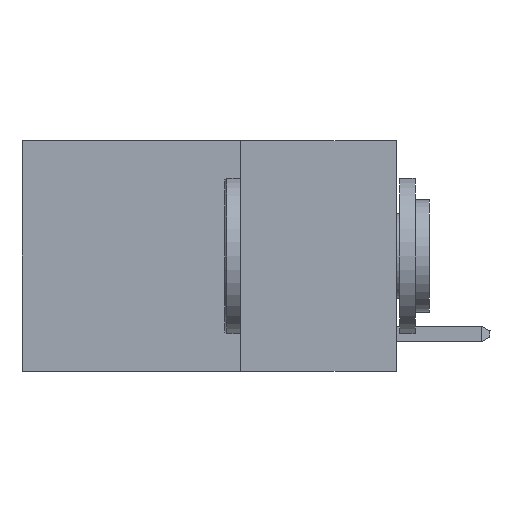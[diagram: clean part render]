
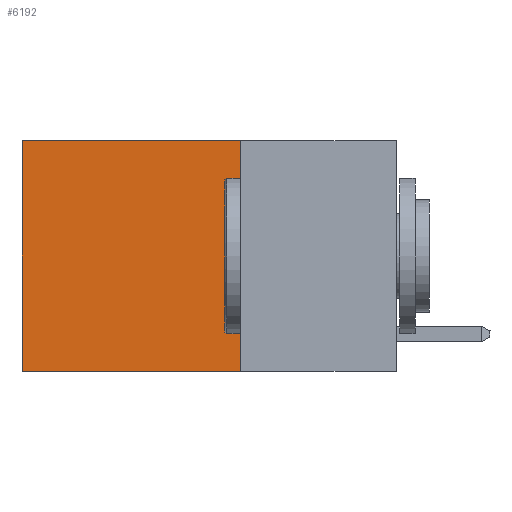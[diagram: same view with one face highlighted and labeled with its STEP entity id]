
A CAD part, left-side view. The second image highlights one B-rep face of the part: STEP entity #6192.
In plain terms, the highlighted planar face has unit normal (-1, 0, 0).
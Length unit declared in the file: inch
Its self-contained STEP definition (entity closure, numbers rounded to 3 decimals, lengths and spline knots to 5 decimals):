
#1 = DIRECTION ( 'NONE',  ( 0., 1., 0. ) ) ;
#405 = CARTESIAN_POINT ( 'NONE',  ( 0.2625, 0.6, 0. ) ) ;
#1059 = DIRECTION ( 'NONE',  ( 0., 0., -1. ) ) ;
#1090 = EDGE_CURVE ( 'NONE', #13211, #1268, #5037, .T. ) ;
#1151 = EDGE_CURVE ( 'NONE', #6891, #13211, #7059, .T. ) ;
#1268 = VERTEX_POINT ( 'NONE', #4481 ) ;
#1320 = ORIENTED_EDGE ( 'NONE', *, *, #17015, .F. ) ;
#2415 = CARTESIAN_POINT ( 'NONE',  ( 0.2625, 0.6, 0. ) ) ;
#2745 = FACE_OUTER_BOUND ( 'NONE', #3893, .T. ) ;
#3444 = CARTESIAN_POINT ( 'NONE',  ( 0.2625, 0.25, -0.37 ) ) ;
#3573 = ORIENTED_EDGE ( 'NONE', *, *, #1090, .T. ) ;
#3893 = EDGE_LOOP ( 'NONE', ( #3573, #12705, #1320, #8097 ) ) ;
#4481 = CARTESIAN_POINT ( 'NONE',  ( 0.2625, 0.6, -0.37 ) ) ;
#4532 = CARTESIAN_POINT ( 'NONE',  ( 0.2625, 0.25, -0.37 ) ) ;
#5037 = LINE ( 'NONE', #2415, #10034 ) ;
#5043 = CARTESIAN_POINT ( 'NONE',  ( 0.2625, 0.25, 0. ) ) ;
#5129 = DIRECTION ( 'NONE',  ( 1., 0., 0. ) ) ;
#5276 = CARTESIAN_POINT ( 'NONE',  ( 0.2625, 0.25, 0. ) ) ;
#5394 = CARTESIAN_POINT ( 'NONE',  ( 0.2625, 0.25, 0. ) ) ;
#6192 = ADVANCED_FACE ( 'NONE', ( #2745 ), #12152, .F. ) ;
#6891 = VERTEX_POINT ( 'NONE', #15689 ) ;
#7059 = LINE ( 'NONE', #5394, #11472 ) ;
#8053 = DIRECTION ( 'NONE',  ( 0., 0., -1. ) ) ;
#8097 = ORIENTED_EDGE ( 'NONE', *, *, #1151, .T. ) ;
#8201 = LINE ( 'NONE', #5276, #11905 ) ;
#10034 = VECTOR ( 'NONE', #8053, 39.37008 ) ;
#10828 = DIRECTION ( 'NONE',  ( 0., 0., -1. ) ) ;
#11129 = DIRECTION ( 'NONE',  ( 0., 1., 0. ) ) ;
#11472 = VECTOR ( 'NONE', #11129, 39.37008 ) ;
#11540 = AXIS2_PLACEMENT_3D ( 'NONE', #5043, #5129, #1059 ) ;
#11905 = VECTOR ( 'NONE', #10828, 39.37008 ) ;
#12152 = PLANE ( 'NONE',  #11540 ) ;
#12289 = EDGE_CURVE ( 'NONE', #14106, #1268, #16965, .T. ) ;
#12705 = ORIENTED_EDGE ( 'NONE', *, *, #12289, .F. ) ;
#13211 = VERTEX_POINT ( 'NONE', #405 ) ;
#14106 = VERTEX_POINT ( 'NONE', #3444 ) ;
#14127 = VECTOR ( 'NONE', #1, 39.37008 ) ;
#15689 = CARTESIAN_POINT ( 'NONE',  ( 0.2625, 0.25, 0. ) ) ;
#16965 = LINE ( 'NONE', #4532, #14127 ) ;
#17015 = EDGE_CURVE ( 'NONE', #6891, #14106, #8201, .T. ) ;
